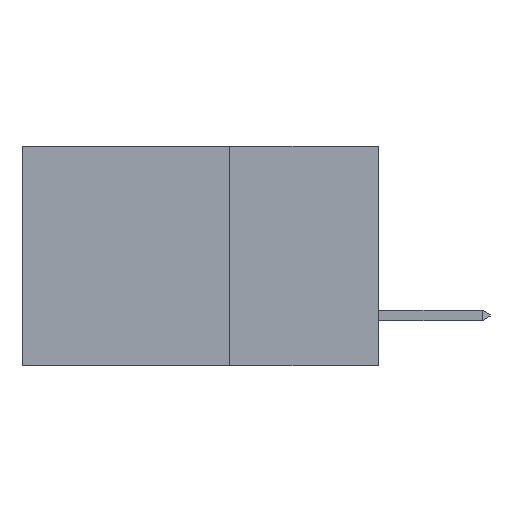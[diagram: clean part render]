
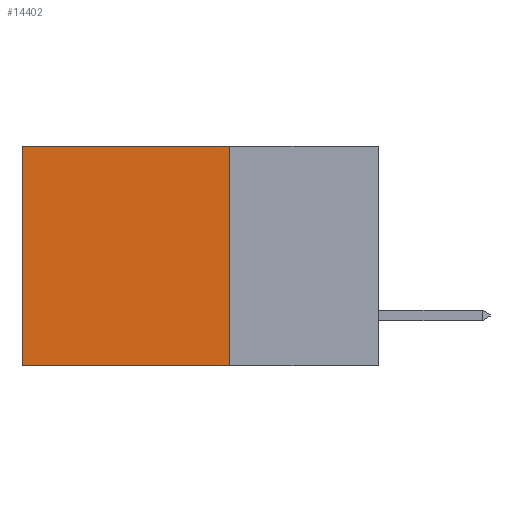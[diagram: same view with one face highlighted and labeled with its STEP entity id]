
A CAD part, left-side view. The second image highlights one B-rep face of the part: STEP entity #14402.
In plain terms, the highlighted planar face has unit normal (-1, 0, 0).
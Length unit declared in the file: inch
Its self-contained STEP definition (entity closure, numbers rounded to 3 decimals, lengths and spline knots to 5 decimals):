
#991 = LINE ( 'NONE', #11226, #14634 ) ;
#1374 = VECTOR ( 'NONE', #15404, 39.37008 ) ;
#1771 = LINE ( 'NONE', #9231, #1374 ) ;
#2659 = CARTESIAN_POINT ( 'NONE',  ( 0.298, 0.6, -0.37 ) ) ;
#3390 = CARTESIAN_POINT ( 'NONE',  ( 0.298, 0.25, 0. ) ) ;
#3574 = CARTESIAN_POINT ( 'NONE',  ( 0.298, 0.6, 0. ) ) ;
#3807 = VERTEX_POINT ( 'NONE', #8183 ) ;
#3963 = AXIS2_PLACEMENT_3D ( 'NONE', #3390, #14883, #7368 ) ;
#4090 = ORIENTED_EDGE ( 'NONE', *, *, #12170, .T. ) ;
#4392 = VERTEX_POINT ( 'NONE', #2659 ) ;
#4769 = EDGE_CURVE ( 'NONE', #7704, #6546, #991, .T. ) ;
#5867 = ORIENTED_EDGE ( 'NONE', *, *, #9124, .T. ) ;
#6010 = DIRECTION ( 'NONE',  ( 0., 1., 0. ) ) ;
#6128 = DIRECTION ( 'NONE',  ( 0., 0., -1. ) ) ;
#6408 = EDGE_LOOP ( 'NONE', ( #5867, #9530, #10486, #4090 ) ) ;
#6546 = VERTEX_POINT ( 'NONE', #10350 ) ;
#7317 = CARTESIAN_POINT ( 'NONE',  ( 0.298, 0.25, -0.37 ) ) ;
#7368 = DIRECTION ( 'NONE',  ( 0., 0., -1. ) ) ;
#7704 = VERTEX_POINT ( 'NONE', #11459 ) ;
#8183 = CARTESIAN_POINT ( 'NONE',  ( 0.298, 0.6, 0. ) ) ;
#8638 = PLANE ( 'NONE',  #3963 ) ;
#8696 = DIRECTION ( 'NONE',  ( 0., 0., -1. ) ) ;
#9059 = EDGE_CURVE ( 'NONE', #6546, #4392, #15590, .T. ) ;
#9124 = EDGE_CURVE ( 'NONE', #3807, #4392, #11533, .T. ) ;
#9135 = FACE_OUTER_BOUND ( 'NONE', #6408, .T. ) ;
#9231 = CARTESIAN_POINT ( 'NONE',  ( 0.298, 0.25, 0. ) ) ;
#9530 = ORIENTED_EDGE ( 'NONE', *, *, #9059, .F. ) ;
#10350 = CARTESIAN_POINT ( 'NONE',  ( 0.298, 0.25, -0.37 ) ) ;
#10486 = ORIENTED_EDGE ( 'NONE', *, *, #4769, .F. ) ;
#11139 = VECTOR ( 'NONE', #6128, 39.37008 ) ;
#11226 = CARTESIAN_POINT ( 'NONE',  ( 0.298, 0.25, 0. ) ) ;
#11459 = CARTESIAN_POINT ( 'NONE',  ( 0.298, 0.25, 0. ) ) ;
#11533 = LINE ( 'NONE', #3574, #11139 ) ;
#12170 = EDGE_CURVE ( 'NONE', #7704, #3807, #1771, .T. ) ;
#12292 = VECTOR ( 'NONE', #6010, 39.37008 ) ;
#14402 = ADVANCED_FACE ( 'NONE', ( #9135 ), #8638, .F. ) ;
#14634 = VECTOR ( 'NONE', #8696, 39.37008 ) ;
#14883 = DIRECTION ( 'NONE',  ( 1., 0., 0. ) ) ;
#15404 = DIRECTION ( 'NONE',  ( 0., 1., 0. ) ) ;
#15590 = LINE ( 'NONE', #7317, #12292 ) ;
